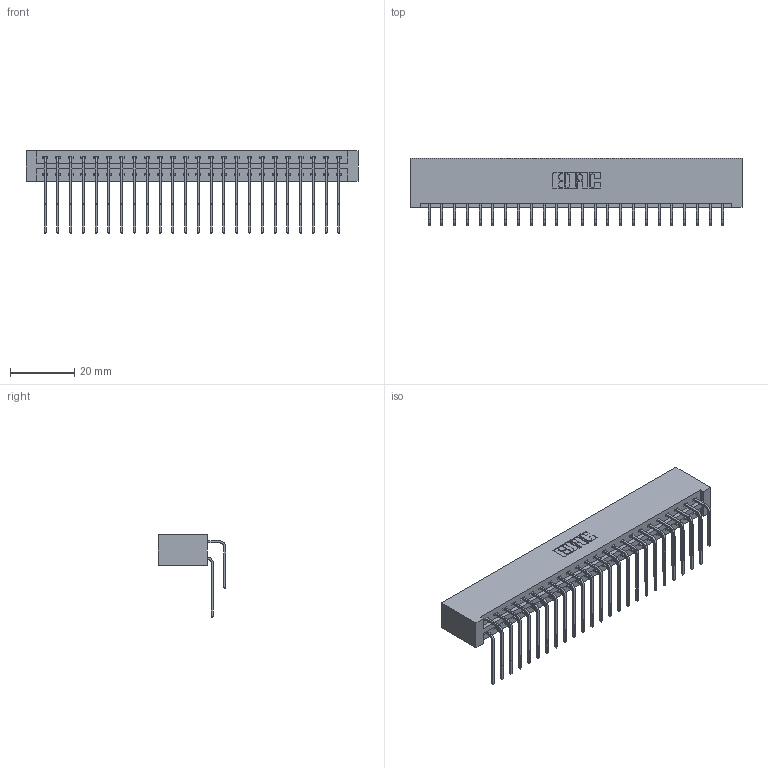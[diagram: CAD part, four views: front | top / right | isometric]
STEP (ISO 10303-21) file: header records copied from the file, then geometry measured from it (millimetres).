
FILE_DESCRIPTION (( 'STEP AP203' ), '1' );
FILE_NAME ('387-048-559-201.STEP', '2019-10-18T10:50:47', ( '' ), ( '' ), 'SwSTEP 2.0', 'SolidWorks 2016', '' );
FILE_SCHEMA (( 'CONFIG_CONTROL_DESIGN' ));
Length unit declared in the file: inch
Products named in the file (4): 345-292-001_559 Tail - 2; 337 Part_No Mounting Lugs; 387-048-559-201; 345-292-001_558 559 Tail - 1
Assembly tree (49 placements, depth 2):
  387-048-559-201
    337 Part_No Mounting Lugs
    345-292-001_558 559 Tail - 1  x24
    345-292-001_559 Tail - 2  x24
Bounding box: 102.97 x 20.9 x 25.53 mm (x, y, z)
Volume: 11650 mm3; surface area: 14442 mm2
Topology: 49 solids, 49 shells, 2794 faces, 8303 edges, 5470 vertices
Faces by surface type: plane 1986, cylinder 808
Entity records: 22443 total; most frequent: CARTESIAN_POINT 3841, ORIENTED_EDGE 3726, DIRECTION 3275, EDGE_CURVE 1863, LINE 1703, VECTOR 1703, VERTEX_POINT 1238, AXIS2_PLACEMENT_3D 786
